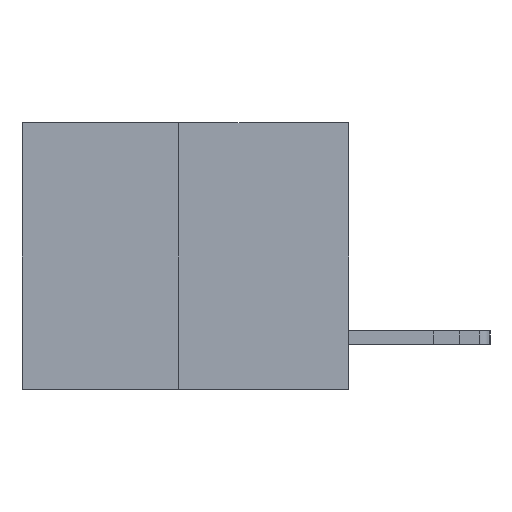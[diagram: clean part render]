
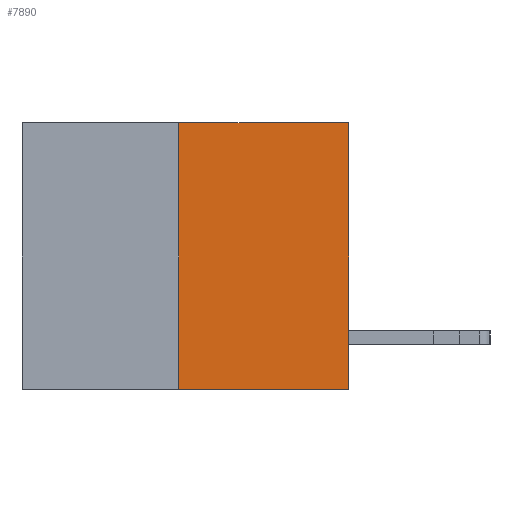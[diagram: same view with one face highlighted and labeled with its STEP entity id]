
A CAD part, left-side view. The second image highlights one B-rep face of the part: STEP entity #7890.
In plain terms, the highlighted planar face has unit normal (-1, 0, 0).
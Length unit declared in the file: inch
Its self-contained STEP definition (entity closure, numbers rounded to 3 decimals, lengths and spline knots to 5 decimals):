
#30 = AXIS2_PLACEMENT_3D ( 'NONE', #18334, #9016, #17252 ) ;
#1693 = VERTEX_POINT ( 'NONE', #19526 ) ;
#2110 = ORIENTED_EDGE ( 'NONE', *, *, #9574, .T. ) ;
#2424 = FACE_OUTER_BOUND ( 'NONE', #18885, .T. ) ;
#2431 = LINE ( 'NONE', #6444, #18421 ) ;
#2488 = EDGE_CURVE ( 'NONE', #4377, #1693, #2431, .T. ) ;
#2637 = DIRECTION ( 'NONE',  ( 0., -1., 0. ) ) ;
#3122 = ORIENTED_EDGE ( 'NONE', *, *, #19568, .F. ) ;
#3361 = VECTOR ( 'NONE', #2637, 39.37008 ) ;
#3675 = CARTESIAN_POINT ( 'NONE',  ( 0., 0., 0. ) ) ;
#4074 = VERTEX_POINT ( 'NONE', #13253 ) ;
#4377 = VERTEX_POINT ( 'NONE', #10042 ) ;
#4698 = VECTOR ( 'NONE', #12900, 39.37008 ) ;
#5730 = CARTESIAN_POINT ( 'NONE',  ( 0., 0.6, 0. ) ) ;
#5779 = VECTOR ( 'NONE', #11267, 39.37008 ) ;
#6444 = CARTESIAN_POINT ( 'NONE',  ( 0., 0.6, -0.49 ) ) ;
#6512 = ORIENTED_EDGE ( 'NONE', *, *, #2488, .T. ) ;
#7890 = ADVANCED_FACE ( 'NONE', ( #2424 ), #12693, .F. ) ;
#8016 = EDGE_CURVE ( 'NONE', #4377, #4074, #9894, .T. ) ;
#9016 = DIRECTION ( 'NONE',  ( 1., 0., 0. ) ) ;
#9574 = EDGE_CURVE ( 'NONE', #1693, #18128, #15631, .T. ) ;
#9894 = LINE ( 'NONE', #9905, #5779 ) ;
#9905 = CARTESIAN_POINT ( 'NONE',  ( 0., 0.312, -0.49 ) ) ;
#9945 = ORIENTED_EDGE ( 'NONE', *, *, #8016, .F. ) ;
#10042 = CARTESIAN_POINT ( 'NONE',  ( 0., 0.312, -0.49 ) ) ;
#11267 = DIRECTION ( 'NONE',  ( 0., 0., 1. ) ) ;
#11629 = LINE ( 'NONE', #5730, #3361 ) ;
#12693 = PLANE ( 'NONE',  #30 ) ;
#12900 = DIRECTION ( 'NONE',  ( 0., 0., 1. ) ) ;
#13253 = CARTESIAN_POINT ( 'NONE',  ( 0., 0.312, 0. ) ) ;
#15631 = LINE ( 'NONE', #3675, #4698 ) ;
#16305 = CARTESIAN_POINT ( 'NONE',  ( 0., 0., 0. ) ) ;
#17252 = DIRECTION ( 'NONE',  ( 0., 0., -1. ) ) ;
#18128 = VERTEX_POINT ( 'NONE', #16305 ) ;
#18334 = CARTESIAN_POINT ( 'NONE',  ( 0., 0.6, 0. ) ) ;
#18421 = VECTOR ( 'NONE', #18785, 39.37008 ) ;
#18785 = DIRECTION ( 'NONE',  ( 0., -1., 0. ) ) ;
#18885 = EDGE_LOOP ( 'NONE', ( #9945, #6512, #2110, #3122 ) ) ;
#19526 = CARTESIAN_POINT ( 'NONE',  ( 0., 0., -0.49 ) ) ;
#19568 = EDGE_CURVE ( 'NONE', #4074, #18128, #11629, .T. ) ;
